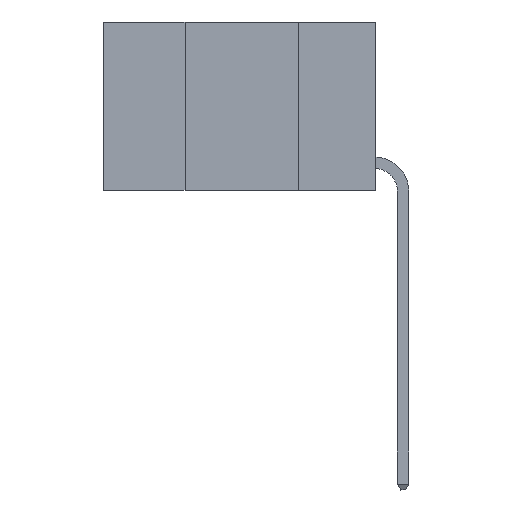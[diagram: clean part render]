
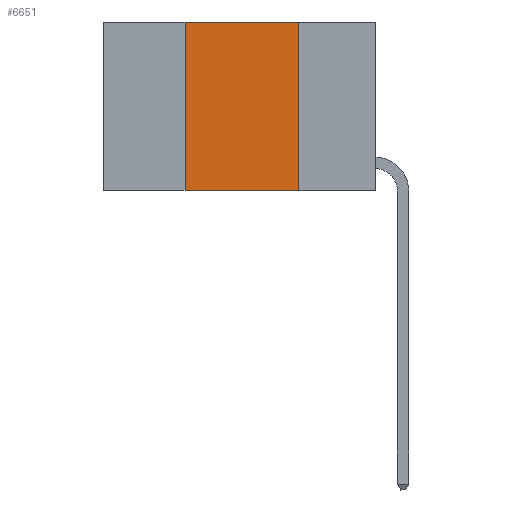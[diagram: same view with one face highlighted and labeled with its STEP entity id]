
A CAD part, left-side view. The second image highlights one B-rep face of the part: STEP entity #6651.
In plain terms, the highlighted planar face has unit normal (-1, 0, 0).
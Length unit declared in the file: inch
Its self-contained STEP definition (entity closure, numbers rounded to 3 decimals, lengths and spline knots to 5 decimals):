
#679 = EDGE_CURVE ( 'NONE', #4943, #8603, #6581, .T. ) ;
#1654 = FACE_OUTER_BOUND ( 'NONE', #10990, .T. ) ;
#2017 = PLANE ( 'NONE',  #9853 ) ;
#3076 = ORIENTED_EDGE ( 'NONE', *, *, #8904, .F. ) ;
#4268 = ORIENTED_EDGE ( 'NONE', *, *, #12667, .F. ) ;
#4467 = CARTESIAN_POINT ( 'NONE',  ( 0., 0.17, -0.37 ) ) ;
#4943 = VERTEX_POINT ( 'NONE', #7600 ) ;
#5719 = CARTESIAN_POINT ( 'NONE',  ( 0., 0.6, 0. ) ) ;
#6472 = VECTOR ( 'NONE', #23240, 39.37008 ) ;
#6581 = LINE ( 'NONE', #19751, #14239 ) ;
#6651 = ADVANCED_FACE ( 'NONE', ( #1654 ), #2017, .F. ) ;
#7600 = CARTESIAN_POINT ( 'NONE',  ( 0., 0.42, -0.37 ) ) ;
#7889 = LINE ( 'NONE', #15398, #16971 ) ;
#7935 = VERTEX_POINT ( 'NONE', #9420 ) ;
#8603 = VERTEX_POINT ( 'NONE', #4467 ) ;
#8904 = EDGE_CURVE ( 'NONE', #22453, #7935, #7889, .T. ) ;
#9239 = ORIENTED_EDGE ( 'NONE', *, *, #679, .T. ) ;
#9420 = CARTESIAN_POINT ( 'NONE',  ( 0., 0.17, 0. ) ) ;
#9853 = AXIS2_PLACEMENT_3D ( 'NONE', #5719, #24268, #22411 ) ;
#10990 = EDGE_LOOP ( 'NONE', ( #14616, #3076, #4268, #9239 ) ) ;
#12667 = EDGE_CURVE ( 'NONE', #4943, #22453, #21417, .T. ) ;
#14239 = VECTOR ( 'NONE', #19627, 39.37008 ) ;
#14616 = ORIENTED_EDGE ( 'NONE', *, *, #18492, .F. ) ;
#14988 = VECTOR ( 'NONE', #18471, 39.37008 ) ;
#15398 = CARTESIAN_POINT ( 'NONE',  ( 0., 0.6, 0. ) ) ;
#16971 = VECTOR ( 'NONE', #22851, 39.37008 ) ;
#18300 = CARTESIAN_POINT ( 'NONE',  ( 0., 0.42, 0. ) ) ;
#18471 = DIRECTION ( 'NONE',  ( 0., 0., -1. ) ) ;
#18492 = EDGE_CURVE ( 'NONE', #7935, #8603, #22716, .T. ) ;
#18712 = CARTESIAN_POINT ( 'NONE',  ( 0., 0.17, 0. ) ) ;
#19105 = CARTESIAN_POINT ( 'NONE',  ( 0., 0.42, 0. ) ) ;
#19627 = DIRECTION ( 'NONE',  ( 0., -1., 0. ) ) ;
#19751 = CARTESIAN_POINT ( 'NONE',  ( 0., 0.6, -0.37 ) ) ;
#21417 = LINE ( 'NONE', #19105, #6472 ) ;
#22411 = DIRECTION ( 'NONE',  ( 0., 0., -1. ) ) ;
#22453 = VERTEX_POINT ( 'NONE', #18300 ) ;
#22716 = LINE ( 'NONE', #18712, #14988 ) ;
#22851 = DIRECTION ( 'NONE',  ( 0., -1., 0. ) ) ;
#23240 = DIRECTION ( 'NONE',  ( 0., 0., 1. ) ) ;
#24268 = DIRECTION ( 'NONE',  ( 1., 0., 0. ) ) ;
